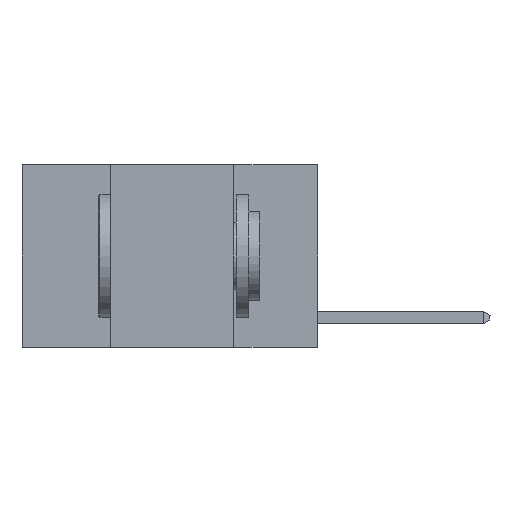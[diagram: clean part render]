
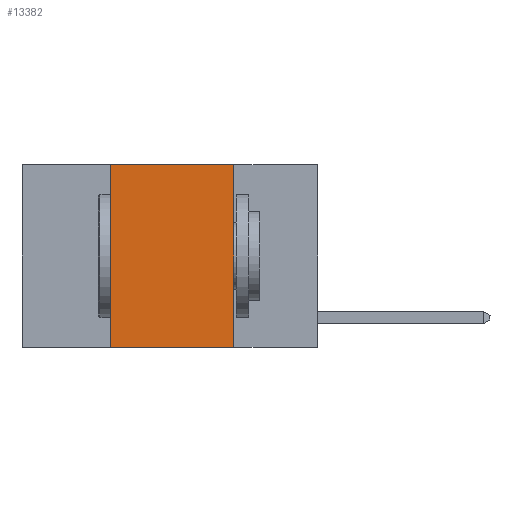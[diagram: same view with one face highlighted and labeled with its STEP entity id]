
A CAD part, left-side view. The second image highlights one B-rep face of the part: STEP entity #13382.
In plain terms, the highlighted planar face has unit normal (-1, 0, 0).
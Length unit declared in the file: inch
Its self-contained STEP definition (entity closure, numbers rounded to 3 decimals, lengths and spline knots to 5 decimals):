
#2028 = CARTESIAN_POINT ( 'NONE',  ( 0., 0.6, -0.37 ) ) ;
#2113 = DIRECTION ( 'NONE',  ( 1., 0., 0. ) ) ;
#2924 = VECTOR ( 'NONE', #9389, 39.37008 ) ;
#3124 = EDGE_CURVE ( 'NONE', #4914, #3733, #8277, .T. ) ;
#3524 = DIRECTION ( 'NONE',  ( 0., 0., -1. ) ) ;
#3733 = VERTEX_POINT ( 'NONE', #4272 ) ;
#4272 = CARTESIAN_POINT ( 'NONE',  ( 0., 0.42, 0. ) ) ;
#4377 = LINE ( 'NONE', #5543, #6391 ) ;
#4559 = CARTESIAN_POINT ( 'NONE',  ( 0., 0.17, 0. ) ) ;
#4573 = FACE_OUTER_BOUND ( 'NONE', #7590, .T. ) ;
#4914 = VERTEX_POINT ( 'NONE', #8258 ) ;
#5543 = CARTESIAN_POINT ( 'NONE',  ( 0., 0.6, 0. ) ) ;
#5654 = EDGE_CURVE ( 'NONE', #12606, #12979, #11378, .T. ) ;
#5729 = VECTOR ( 'NONE', #9459, 39.37008 ) ;
#6391 = VECTOR ( 'NONE', #10373, 39.37008 ) ;
#7590 = EDGE_LOOP ( 'NONE', ( #9660, #12159, #15385, #12632 ) ) ;
#8056 = LINE ( 'NONE', #2028, #14647 ) ;
#8258 = CARTESIAN_POINT ( 'NONE',  ( 0., 0.42, -0.37 ) ) ;
#8277 = LINE ( 'NONE', #12999, #5729 ) ;
#9024 = EDGE_CURVE ( 'NONE', #4914, #12979, #8056, .T. ) ;
#9383 = CARTESIAN_POINT ( 'NONE',  ( 0., 0.17, 0. ) ) ;
#9389 = DIRECTION ( 'NONE',  ( 0., 0., -1. ) ) ;
#9459 = DIRECTION ( 'NONE',  ( 0., 0., 1. ) ) ;
#9660 = ORIENTED_EDGE ( 'NONE', *, *, #5654, .F. ) ;
#10373 = DIRECTION ( 'NONE',  ( 0., -1., 0. ) ) ;
#10933 = AXIS2_PLACEMENT_3D ( 'NONE', #11765, #2113, #3524 ) ;
#11180 = EDGE_CURVE ( 'NONE', #3733, #12606, #4377, .T. ) ;
#11378 = LINE ( 'NONE', #4559, #2924 ) ;
#11652 = CARTESIAN_POINT ( 'NONE',  ( 0., 0.17, -0.37 ) ) ;
#11684 = DIRECTION ( 'NONE',  ( 0., -1., 0. ) ) ;
#11765 = CARTESIAN_POINT ( 'NONE',  ( 0., 0.6, 0. ) ) ;
#11915 = PLANE ( 'NONE',  #10933 ) ;
#12159 = ORIENTED_EDGE ( 'NONE', *, *, #11180, .F. ) ;
#12606 = VERTEX_POINT ( 'NONE', #9383 ) ;
#12632 = ORIENTED_EDGE ( 'NONE', *, *, #9024, .T. ) ;
#12979 = VERTEX_POINT ( 'NONE', #11652 ) ;
#12999 = CARTESIAN_POINT ( 'NONE',  ( 0., 0.42, 0. ) ) ;
#13382 = ADVANCED_FACE ( 'NONE', ( #4573 ), #11915, .F. ) ;
#14647 = VECTOR ( 'NONE', #11684, 39.37008 ) ;
#15385 = ORIENTED_EDGE ( 'NONE', *, *, #3124, .F. ) ;
